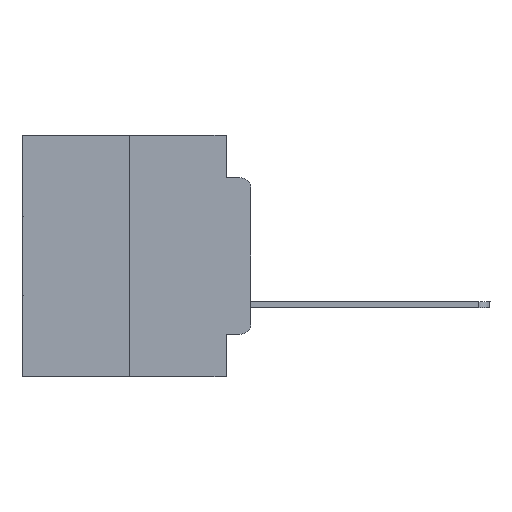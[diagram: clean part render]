
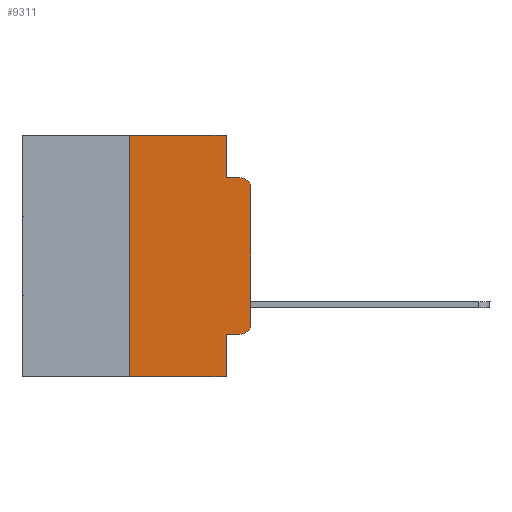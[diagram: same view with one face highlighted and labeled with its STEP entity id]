
A CAD part, left-side view. The second image highlights one B-rep face of the part: STEP entity #9311.
In plain terms, the highlighted planar face has unit normal (-1, 0, 0).
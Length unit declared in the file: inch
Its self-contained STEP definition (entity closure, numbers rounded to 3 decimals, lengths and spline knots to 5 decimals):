
#1032 = VERTEX_POINT ( 'NONE', #10381 ) ;
#1162 = DIRECTION ( 'NONE',  ( -1., 0., 0. ) ) ;
#1355 = EDGE_CURVE ( 'NONE', #1032, #14196, #24489, .T. ) ;
#1841 = ORIENTED_EDGE ( 'NONE', *, *, #6517, .F. ) ;
#1961 = CARTESIAN_POINT ( 'NONE',  ( 0., 0.051, 0. ) ) ;
#1983 = DIRECTION ( 'NONE',  ( 0., 0., -1. ) ) ;
#3308 = VERTEX_POINT ( 'NONE', #29327 ) ;
#3358 = FACE_OUTER_BOUND ( 'NONE', #27695, .T. ) ;
#3383 = CARTESIAN_POINT ( 'NONE',  ( 0., 0., -0.3915 ) ) ;
#3869 = LINE ( 'NONE', #5298, #22658 ) ;
#4349 = DIRECTION ( 'NONE',  ( 0., 0., -1. ) ) ;
#4686 = DIRECTION ( 'NONE',  ( 0., -1., 0. ) ) ;
#4748 = ORIENTED_EDGE ( 'NONE', *, *, #26218, .T. ) ;
#4832 = EDGE_CURVE ( 'NONE', #29256, #6658, #20553, .T. ) ;
#5111 = EDGE_CURVE ( 'NONE', #14196, #14724, #29028, .T. ) ;
#5298 = CARTESIAN_POINT ( 'NONE',  ( 0., 0.051, -0.0885 ) ) ;
#5562 = VECTOR ( 'NONE', #4686, 39.37008 ) ;
#6321 = CARTESIAN_POINT ( 'NONE',  ( 0., 0.051, -0.0885 ) ) ;
#6517 = EDGE_CURVE ( 'NONE', #20353, #1032, #15642, .T. ) ;
#6658 = VERTEX_POINT ( 'NONE', #26870 ) ;
#7249 = CARTESIAN_POINT ( 'NONE',  ( 0., 0.473, -0.5 ) ) ;
#7703 = ORIENTED_EDGE ( 'NONE', *, *, #14264, .F. ) ;
#7716 = VECTOR ( 'NONE', #20002, 39.37008 ) ;
#7914 = EDGE_CURVE ( 'NONE', #13316, #16475, #15222, .T. ) ;
#8587 = AXIS2_PLACEMENT_3D ( 'NONE', #19690, #14937, #10320 ) ;
#9311 = ADVANCED_FACE ( 'NONE', ( #3358 ), #23217, .F. ) ;
#9421 = EDGE_CURVE ( 'NONE', #20353, #6658, #12548, .T. ) ;
#9473 = VECTOR ( 'NONE', #4349, 39.37008 ) ;
#9521 = CARTESIAN_POINT ( 'NONE',  ( 0., 0.473, 0. ) ) ;
#9893 = LINE ( 'NONE', #19366, #23177 ) ;
#10320 = DIRECTION ( 'NONE',  ( 0., 0., -1. ) ) ;
#10381 = CARTESIAN_POINT ( 'NONE',  ( 0., 0.25, 0. ) ) ;
#10398 = ORIENTED_EDGE ( 'NONE', *, *, #7914, .T. ) ;
#10642 = CARTESIAN_POINT ( 'NONE',  ( 0., 0.02, -0.1085 ) ) ;
#11573 = DIRECTION ( 'NONE',  ( 1., 0., 0. ) ) ;
#11811 = ORIENTED_EDGE ( 'NONE', *, *, #19343, .T. ) ;
#11838 = ORIENTED_EDGE ( 'NONE', *, *, #9421, .T. ) ;
#12282 = VECTOR ( 'NONE', #30450, 39.37008 ) ;
#12475 = CARTESIAN_POINT ( 'NONE',  ( 0., 0.051, 0. ) ) ;
#12548 = LINE ( 'NONE', #7249, #5562 ) ;
#12610 = ORIENTED_EDGE ( 'NONE', *, *, #4832, .F. ) ;
#12994 = CARTESIAN_POINT ( 'NONE',  ( 0., 0.051, -0.4115 ) ) ;
#13316 = VERTEX_POINT ( 'NONE', #28640 ) ;
#13536 = VECTOR ( 'NONE', #1983, 39.37008 ) ;
#13573 = ORIENTED_EDGE ( 'NONE', *, *, #1355, .F. ) ;
#13595 = CARTESIAN_POINT ( 'NONE',  ( 0., 0.051, 0. ) ) ;
#14138 = CARTESIAN_POINT ( 'NONE',  ( 0., 0.051, -0.4115 ) ) ;
#14196 = VERTEX_POINT ( 'NONE', #12475 ) ;
#14264 = EDGE_CURVE ( 'NONE', #14724, #16475, #3869, .T. ) ;
#14281 = AXIS2_PLACEMENT_3D ( 'NONE', #30211, #11573, #28061 ) ;
#14405 = DIRECTION ( 'NONE',  ( 0., 0., 1. ) ) ;
#14724 = VERTEX_POINT ( 'NONE', #6321 ) ;
#14767 = ORIENTED_EDGE ( 'NONE', *, *, #25807, .T. ) ;
#14937 = DIRECTION ( 'NONE',  ( -1., 0., 0. ) ) ;
#15222 = CIRCLE ( 'NONE', #27510, 0.02 ) ;
#15277 = VECTOR ( 'NONE', #14405, 39.37008 ) ;
#15642 = LINE ( 'NONE', #26397, #15277 ) ;
#16215 = CIRCLE ( 'NONE', #8587, 0.02 ) ;
#16475 = VERTEX_POINT ( 'NONE', #28729 ) ;
#19343 = EDGE_CURVE ( 'NONE', #3308, #23097, #16215, .T. ) ;
#19366 = CARTESIAN_POINT ( 'NONE',  ( 0., 0., 0. ) ) ;
#19690 = CARTESIAN_POINT ( 'NONE',  ( 0., 0.02, -0.3915 ) ) ;
#20002 = DIRECTION ( 'NONE',  ( 0., -1., 0. ) ) ;
#20353 = VERTEX_POINT ( 'NONE', #29219 ) ;
#20553 = LINE ( 'NONE', #13595, #13536 ) ;
#21435 = DIRECTION ( 'NONE',  ( 0., -1., 0. ) ) ;
#22658 = VECTOR ( 'NONE', #21435, 39.37008 ) ;
#22820 = LINE ( 'NONE', #12994, #7716 ) ;
#23097 = VERTEX_POINT ( 'NONE', #3383 ) ;
#23177 = VECTOR ( 'NONE', #28549, 39.37008 ) ;
#23217 = PLANE ( 'NONE',  #14281 ) ;
#24489 = LINE ( 'NONE', #9521, #12282 ) ;
#24499 = ORIENTED_EDGE ( 'NONE', *, *, #5111, .F. ) ;
#25807 = EDGE_CURVE ( 'NONE', #29256, #3308, #22820, .T. ) ;
#26218 = EDGE_CURVE ( 'NONE', #23097, #13316, #9893, .T. ) ;
#26397 = CARTESIAN_POINT ( 'NONE',  ( 0., 0.25, 0. ) ) ;
#26870 = CARTESIAN_POINT ( 'NONE',  ( 0., 0.051, -0.5 ) ) ;
#27428 = DIRECTION ( 'NONE',  ( 0., 0., -1. ) ) ;
#27510 = AXIS2_PLACEMENT_3D ( 'NONE', #10642, #1162, #27428 ) ;
#27695 = EDGE_LOOP ( 'NONE', ( #4748, #10398, #7703, #24499, #13573, #1841, #11838, #12610, #14767, #11811 ) ) ;
#28061 = DIRECTION ( 'NONE',  ( 0., 0., -1. ) ) ;
#28549 = DIRECTION ( 'NONE',  ( 0., 0., 1. ) ) ;
#28640 = CARTESIAN_POINT ( 'NONE',  ( 0., 0., -0.1085 ) ) ;
#28729 = CARTESIAN_POINT ( 'NONE',  ( 0., 0.02, -0.0885 ) ) ;
#29028 = LINE ( 'NONE', #1961, #9473 ) ;
#29219 = CARTESIAN_POINT ( 'NONE',  ( 0., 0.25, -0.5 ) ) ;
#29256 = VERTEX_POINT ( 'NONE', #14138 ) ;
#29327 = CARTESIAN_POINT ( 'NONE',  ( 0., 0.02, -0.4115 ) ) ;
#30211 = CARTESIAN_POINT ( 'NONE',  ( 0., 0.473, 0. ) ) ;
#30450 = DIRECTION ( 'NONE',  ( 0., -1., 0. ) ) ;
